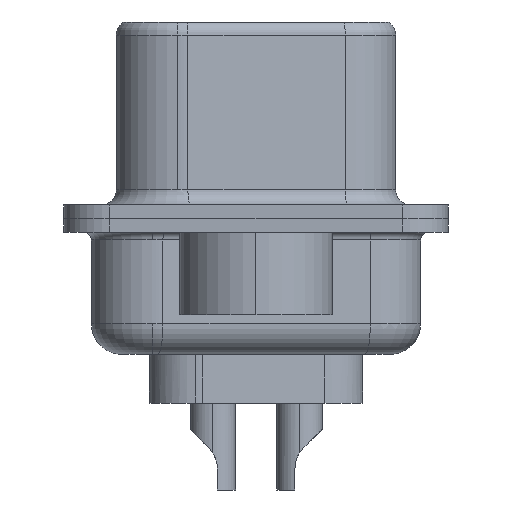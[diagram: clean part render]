
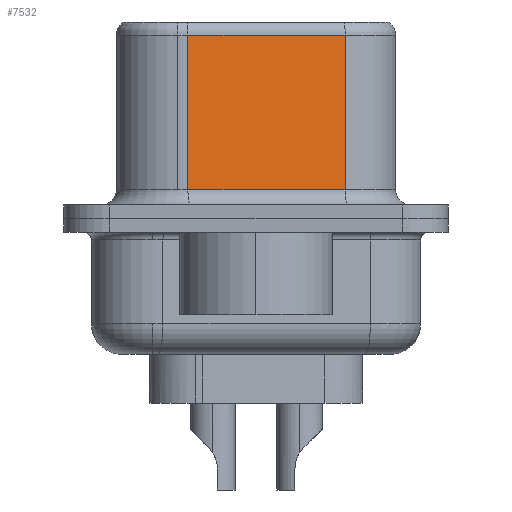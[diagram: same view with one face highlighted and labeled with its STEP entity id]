
A CAD part, left-side view. The second image highlights one B-rep face of the part: STEP entity #7532.
In plain terms, the highlighted planar face has unit normal (-0.985, -0.174, 0).
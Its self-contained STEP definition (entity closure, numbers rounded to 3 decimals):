
#332 = PLANE ( 'NONE',  #15279 ) ;
#497 = EDGE_CURVE ( 'NONE', #2586, #1184, #5178, .T. ) ;
#850 = LINE ( 'NONE', #3798, #7115 ) ;
#1097 = VECTOR ( 'NONE', #4690, 1000. ) ;
#1184 = VERTEX_POINT ( 'NONE', #13711 ) ;
#2586 = VERTEX_POINT ( 'NONE', #3672 ) ;
#2922 = LINE ( 'NONE', #2994, #15772 ) ;
#2994 = CARTESIAN_POINT ( 'NONE',  ( 3.665, 2.233, 6.52 ) ) ;
#3672 = CARTESIAN_POINT ( 'NONE',  ( 4.575, -2.927, 6.02 ) ) ;
#3798 = CARTESIAN_POINT ( 'NONE',  ( 4.575, -2.927, 0.95 ) ) ;
#3857 = EDGE_LOOP ( 'NONE', ( #4810, #7214, #6646, #14143 ) ) ;
#4070 = LINE ( 'NONE', #15916, #1097 ) ;
#4239 = DIRECTION ( 'NONE',  ( 0., 0., -1. ) ) ;
#4430 = VECTOR ( 'NONE', #14774, 1000. ) ;
#4446 = CARTESIAN_POINT ( 'NONE',  ( 3.665, 2.233, 0.95 ) ) ;
#4690 = DIRECTION ( 'NONE',  ( -0.174, 0.985, 0. ) ) ;
#4810 = ORIENTED_EDGE ( 'NONE', *, *, #497, .F. ) ;
#5178 = LINE ( 'NONE', #14057, #4430 ) ;
#6646 = ORIENTED_EDGE ( 'NONE', *, *, #12075, .T. ) ;
#6648 = DIRECTION ( 'NONE',  ( -0.174, 0.985, 0. ) ) ;
#6785 = CARTESIAN_POINT ( 'NONE',  ( 3.665, 2.233, 6.02 ) ) ;
#7002 = VERTEX_POINT ( 'NONE', #4446 ) ;
#7115 = VECTOR ( 'NONE', #13758, 1000. ) ;
#7214 = ORIENTED_EDGE ( 'NONE', *, *, #13981, .T. ) ;
#7532 = ADVANCED_FACE ( 'NONE', ( #11672 ), #332, .F. ) ;
#10273 = VERTEX_POINT ( 'NONE', #6785 ) ;
#11573 = CARTESIAN_POINT ( 'NONE',  ( 4.575, -2.927, 6.52 ) ) ;
#11672 = FACE_OUTER_BOUND ( 'NONE', #3857, .T. ) ;
#12075 = EDGE_CURVE ( 'NONE', #10273, #7002, #2922, .T. ) ;
#13711 = CARTESIAN_POINT ( 'NONE',  ( 4.575, -2.927, 0.95 ) ) ;
#13758 = DIRECTION ( 'NONE',  ( 0.174, -0.985, 0. ) ) ;
#13981 = EDGE_CURVE ( 'NONE', #2586, #10273, #4070, .T. ) ;
#14057 = CARTESIAN_POINT ( 'NONE',  ( 4.575, -2.927, 6.52 ) ) ;
#14128 = DIRECTION ( 'NONE',  ( 0.985, 0.174, 0. ) ) ;
#14143 = ORIENTED_EDGE ( 'NONE', *, *, #15376, .T. ) ;
#14774 = DIRECTION ( 'NONE',  ( 0., 0., -1. ) ) ;
#15279 = AXIS2_PLACEMENT_3D ( 'NONE', #11573, #14128, #6648 ) ;
#15376 = EDGE_CURVE ( 'NONE', #7002, #1184, #850, .T. ) ;
#15772 = VECTOR ( 'NONE', #4239, 1000. ) ;
#15916 = CARTESIAN_POINT ( 'NONE',  ( 4.575, -2.927, 6.02 ) ) ;
